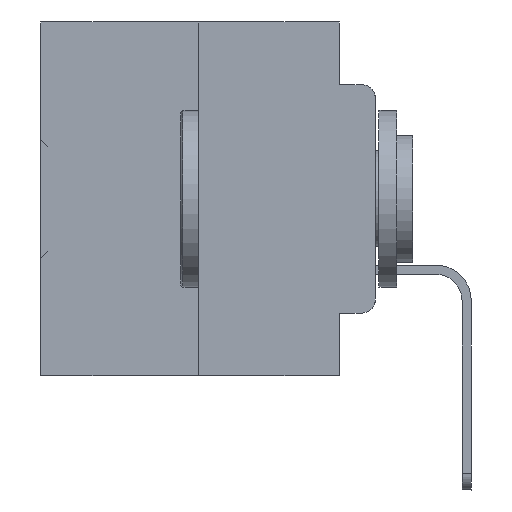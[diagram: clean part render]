
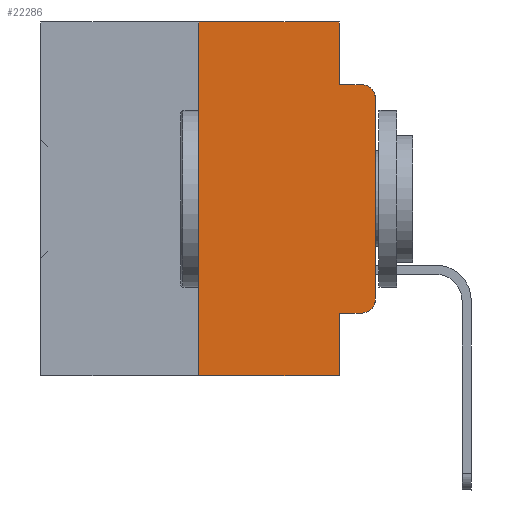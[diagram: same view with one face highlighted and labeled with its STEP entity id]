
A CAD part, left-side view. The second image highlights one B-rep face of the part: STEP entity #22286.
In plain terms, the highlighted planar face has unit normal (-1, 0, 0).
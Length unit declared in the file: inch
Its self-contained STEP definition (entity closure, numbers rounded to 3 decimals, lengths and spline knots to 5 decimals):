
#203 = CIRCLE ( 'NONE', #12697, 0.02 ) ;
#218 = VECTOR ( 'NONE', #7251, 39.37008 ) ;
#379 = DIRECTION ( 'NONE',  ( 0., -1., 0. ) ) ;
#452 = EDGE_CURVE ( 'NONE', #23599, #24163, #10211, .T. ) ;
#551 = EDGE_CURVE ( 'NONE', #9647, #32688, #2722, .T. ) ;
#614 = EDGE_CURVE ( 'NONE', #23599, #6790, #14371, .T. ) ;
#689 = CARTESIAN_POINT ( 'NONE',  ( 0., 0.051, -0.5 ) ) ;
#729 = CIRCLE ( 'NONE', #4926, 0.02 ) ;
#2201 = CARTESIAN_POINT ( 'NONE',  ( 0., 0.473, 0. ) ) ;
#2722 = LINE ( 'NONE', #29839, #5544 ) ;
#2872 = CARTESIAN_POINT ( 'NONE',  ( 0., 0.051, -0.4115 ) ) ;
#3480 = ORIENTED_EDGE ( 'NONE', *, *, #28358, .F. ) ;
#3717 = VECTOR ( 'NONE', #22749, 39.37008 ) ;
#4631 = CARTESIAN_POINT ( 'NONE',  ( 0., 0.25, 0. ) ) ;
#4926 = AXIS2_PLACEMENT_3D ( 'NONE', #13166, #33604, #16031 ) ;
#5544 = VECTOR ( 'NONE', #18253, 39.37008 ) ;
#5809 = AXIS2_PLACEMENT_3D ( 'NONE', #2201, #8095, #23202 ) ;
#6042 = ORIENTED_EDGE ( 'NONE', *, *, #30594, .F. ) ;
#6319 = CARTESIAN_POINT ( 'NONE',  ( 0., 0.02, -0.0885 ) ) ;
#6790 = VERTEX_POINT ( 'NONE', #16008 ) ;
#7251 = DIRECTION ( 'NONE',  ( 0., -1., 0. ) ) ;
#8095 = DIRECTION ( 'NONE',  ( 1., 0., 0. ) ) ;
#9647 = VERTEX_POINT ( 'NONE', #19914 ) ;
#10211 = LINE ( 'NONE', #32487, #30229 ) ;
#11992 = CARTESIAN_POINT ( 'NONE',  ( 0., 0.02, -0.3915 ) ) ;
#12615 = DIRECTION ( 'NONE',  ( 0., 0., 1. ) ) ;
#12697 = AXIS2_PLACEMENT_3D ( 'NONE', #11992, #38548, #14465 ) ;
#13125 = LINE ( 'NONE', #23009, #30806 ) ;
#13166 = CARTESIAN_POINT ( 'NONE',  ( 0., 0.02, -0.1085 ) ) ;
#14232 = LINE ( 'NONE', #31463, #218 ) ;
#14371 = LINE ( 'NONE', #2872, #22277 ) ;
#14465 = DIRECTION ( 'NONE',  ( 0., 0., -1. ) ) ;
#14472 = LINE ( 'NONE', #34851, #3717 ) ;
#15165 = VERTEX_POINT ( 'NONE', #30854 ) ;
#15235 = EDGE_LOOP ( 'NONE', ( #27488, #36236, #16052, #36072, #6042, #3480, #34073, #30414, #26655, #24448 ) ) ;
#16008 = CARTESIAN_POINT ( 'NONE',  ( 0., 0.02, -0.4115 ) ) ;
#16031 = DIRECTION ( 'NONE',  ( 0., 0., -1. ) ) ;
#16052 = ORIENTED_EDGE ( 'NONE', *, *, #23840, .F. ) ;
#16219 = VERTEX_POINT ( 'NONE', #6319 ) ;
#16255 = VECTOR ( 'NONE', #12615, 39.37008 ) ;
#18253 = DIRECTION ( 'NONE',  ( 0., 0., -1. ) ) ;
#18313 = EDGE_CURVE ( 'NONE', #22141, #16219, #729, .T. ) ;
#19133 = EDGE_CURVE ( 'NONE', #6790, #24619, #203, .T. ) ;
#19626 = VERTEX_POINT ( 'NONE', #4631 ) ;
#19914 = CARTESIAN_POINT ( 'NONE',  ( 0., 0.051, 0. ) ) ;
#20347 = DIRECTION ( 'NONE',  ( 0., 0., -1. ) ) ;
#21833 = CARTESIAN_POINT ( 'NONE',  ( 0., 0.051, -0.0885 ) ) ;
#22141 = VERTEX_POINT ( 'NONE', #25604 ) ;
#22277 = VECTOR ( 'NONE', #379, 39.37008 ) ;
#22286 = ADVANCED_FACE ( 'NONE', ( #31930 ), #34789, .F. ) ;
#22749 = DIRECTION ( 'NONE',  ( 0., -1., 0. ) ) ;
#23009 = CARTESIAN_POINT ( 'NONE',  ( 0., 0.051, -0.0885 ) ) ;
#23202 = DIRECTION ( 'NONE',  ( 0., 0., -1. ) ) ;
#23599 = VERTEX_POINT ( 'NONE', #26662 ) ;
#23840 = EDGE_CURVE ( 'NONE', #32688, #16219, #13125, .T. ) ;
#24163 = VERTEX_POINT ( 'NONE', #689 ) ;
#24448 = ORIENTED_EDGE ( 'NONE', *, *, #19133, .T. ) ;
#24619 = VERTEX_POINT ( 'NONE', #35720 ) ;
#25604 = CARTESIAN_POINT ( 'NONE',  ( 0., 0., -0.1085 ) ) ;
#26655 = ORIENTED_EDGE ( 'NONE', *, *, #614, .T. ) ;
#26662 = CARTESIAN_POINT ( 'NONE',  ( 0., 0.051, -0.4115 ) ) ;
#27488 = ORIENTED_EDGE ( 'NONE', *, *, #29406, .T. ) ;
#28358 = EDGE_CURVE ( 'NONE', #15165, #19626, #32114, .T. ) ;
#29175 = VECTOR ( 'NONE', #35723, 39.37008 ) ;
#29406 = EDGE_CURVE ( 'NONE', #24619, #22141, #38041, .T. ) ;
#29839 = CARTESIAN_POINT ( 'NONE',  ( 0., 0.051, 0. ) ) ;
#30229 = VECTOR ( 'NONE', #20347, 39.37008 ) ;
#30414 = ORIENTED_EDGE ( 'NONE', *, *, #452, .F. ) ;
#30594 = EDGE_CURVE ( 'NONE', #19626, #9647, #14472, .T. ) ;
#30686 = CARTESIAN_POINT ( 'NONE',  ( 0., 0.25, 0. ) ) ;
#30806 = VECTOR ( 'NONE', #35131, 39.37008 ) ;
#30854 = CARTESIAN_POINT ( 'NONE',  ( 0., 0.25, -0.5 ) ) ;
#31463 = CARTESIAN_POINT ( 'NONE',  ( 0., 0.473, -0.5 ) ) ;
#31930 = FACE_OUTER_BOUND ( 'NONE', #15235, .T. ) ;
#32114 = LINE ( 'NONE', #30686, #16255 ) ;
#32487 = CARTESIAN_POINT ( 'NONE',  ( 0., 0.051, 0. ) ) ;
#32688 = VERTEX_POINT ( 'NONE', #21833 ) ;
#33604 = DIRECTION ( 'NONE',  ( -1., 0., 0. ) ) ;
#34073 = ORIENTED_EDGE ( 'NONE', *, *, #36578, .T. ) ;
#34789 = PLANE ( 'NONE',  #5809 ) ;
#34851 = CARTESIAN_POINT ( 'NONE',  ( 0., 0.473, 0. ) ) ;
#35131 = DIRECTION ( 'NONE',  ( 0., -1., 0. ) ) ;
#35720 = CARTESIAN_POINT ( 'NONE',  ( 0., 0., -0.3915 ) ) ;
#35723 = DIRECTION ( 'NONE',  ( 0., 0., 1. ) ) ;
#36072 = ORIENTED_EDGE ( 'NONE', *, *, #551, .F. ) ;
#36236 = ORIENTED_EDGE ( 'NONE', *, *, #18313, .T. ) ;
#36578 = EDGE_CURVE ( 'NONE', #15165, #24163, #14232, .T. ) ;
#38041 = LINE ( 'NONE', #38326, #29175 ) ;
#38326 = CARTESIAN_POINT ( 'NONE',  ( 0., 0., 0. ) ) ;
#38548 = DIRECTION ( 'NONE',  ( -1., 0., 0. ) ) ;
